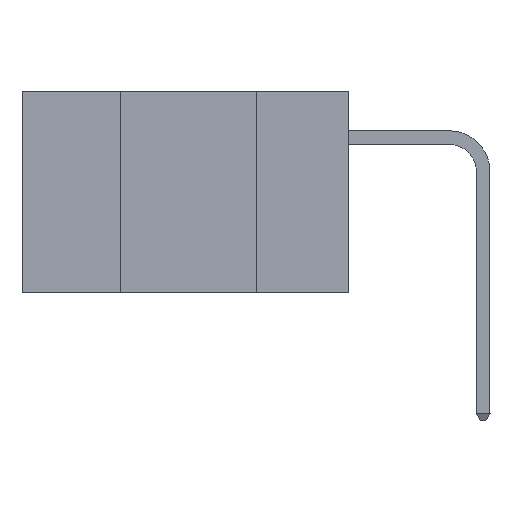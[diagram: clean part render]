
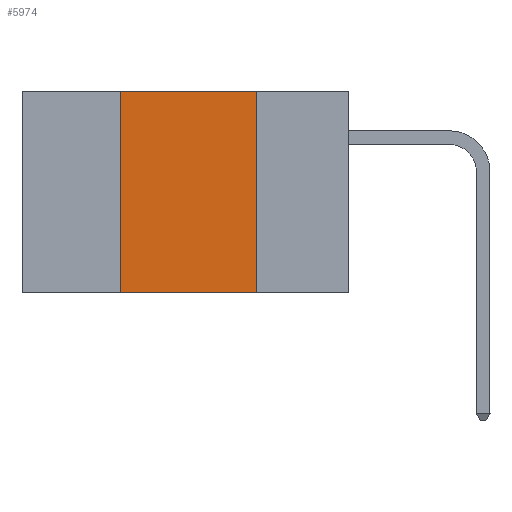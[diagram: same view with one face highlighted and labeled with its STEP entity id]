
A CAD part, left-side view. The second image highlights one B-rep face of the part: STEP entity #5974.
In plain terms, the highlighted planar face has unit normal (-1, 0, 0).
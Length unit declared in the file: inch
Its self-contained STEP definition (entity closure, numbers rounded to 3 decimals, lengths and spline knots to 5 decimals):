
#44 = LINE ( 'NONE', #31391, #395 ) ;
#395 = VECTOR ( 'NONE', #35754, 39.37008 ) ;
#605 = DIRECTION ( 'NONE',  ( 0., 0., 1. ) ) ;
#1718 = FACE_OUTER_BOUND ( 'NONE', #8582, .T. ) ;
#2765 = CARTESIAN_POINT ( 'NONE',  ( 0., 0.17, 0. ) ) ;
#5562 = DIRECTION ( 'NONE',  ( 0., 0., -1. ) ) ;
#5974 = ADVANCED_FACE ( 'NONE', ( #1718 ), #33553, .F. ) ;
#7809 = CARTESIAN_POINT ( 'NONE',  ( 0., 0.42, 0. ) ) ;
#8582 = EDGE_LOOP ( 'NONE', ( #48907, #44903, #46629, #34374 ) ) ;
#10178 = DIRECTION ( 'NONE',  ( 1., 0., 0. ) ) ;
#10410 = VERTEX_POINT ( 'NONE', #21511 ) ;
#11070 = EDGE_CURVE ( 'NONE', #30734, #27353, #47116, .T. ) ;
#11630 = AXIS2_PLACEMENT_3D ( 'NONE', #28947, #10178, #5562 ) ;
#11685 = EDGE_CURVE ( 'NONE', #30734, #18602, #44, .T. ) ;
#15844 = EDGE_CURVE ( 'NONE', #10410, #18602, #25643, .T. ) ;
#16473 = VECTOR ( 'NONE', #39250, 39.37008 ) ;
#18415 = DIRECTION ( 'NONE',  ( 0., 0., -1. ) ) ;
#18602 = VERTEX_POINT ( 'NONE', #47505 ) ;
#21511 = CARTESIAN_POINT ( 'NONE',  ( 0., 0.17, 0. ) ) ;
#23012 = CARTESIAN_POINT ( 'NONE',  ( 0., 0.42, -0.37 ) ) ;
#25643 = LINE ( 'NONE', #2765, #50041 ) ;
#27353 = VERTEX_POINT ( 'NONE', #28538 ) ;
#28538 = CARTESIAN_POINT ( 'NONE',  ( 0., 0.42, 0. ) ) ;
#28947 = CARTESIAN_POINT ( 'NONE',  ( 0., 0.6, 0. ) ) ;
#30734 = VERTEX_POINT ( 'NONE', #23012 ) ;
#31391 = CARTESIAN_POINT ( 'NONE',  ( 0., 0.6, -0.37 ) ) ;
#32750 = EDGE_CURVE ( 'NONE', #27353, #10410, #38994, .T. ) ;
#33553 = PLANE ( 'NONE',  #11630 ) ;
#34374 = ORIENTED_EDGE ( 'NONE', *, *, #11685, .T. ) ;
#35754 = DIRECTION ( 'NONE',  ( 0., -1., 0. ) ) ;
#38475 = CARTESIAN_POINT ( 'NONE',  ( 0., 0.6, 0. ) ) ;
#38994 = LINE ( 'NONE', #38475, #16473 ) ;
#39250 = DIRECTION ( 'NONE',  ( 0., -1., 0. ) ) ;
#44903 = ORIENTED_EDGE ( 'NONE', *, *, #32750, .F. ) ;
#46629 = ORIENTED_EDGE ( 'NONE', *, *, #11070, .F. ) ;
#47116 = LINE ( 'NONE', #7809, #48786 ) ;
#47505 = CARTESIAN_POINT ( 'NONE',  ( 0., 0.17, -0.37 ) ) ;
#48786 = VECTOR ( 'NONE', #605, 39.37008 ) ;
#48907 = ORIENTED_EDGE ( 'NONE', *, *, #15844, .F. ) ;
#50041 = VECTOR ( 'NONE', #18415, 39.37008 ) ;
